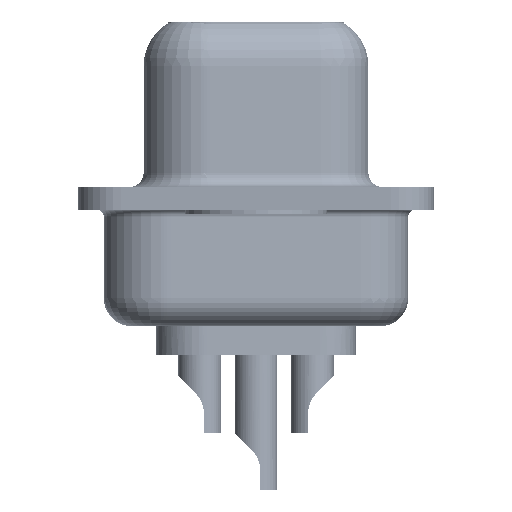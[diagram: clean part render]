
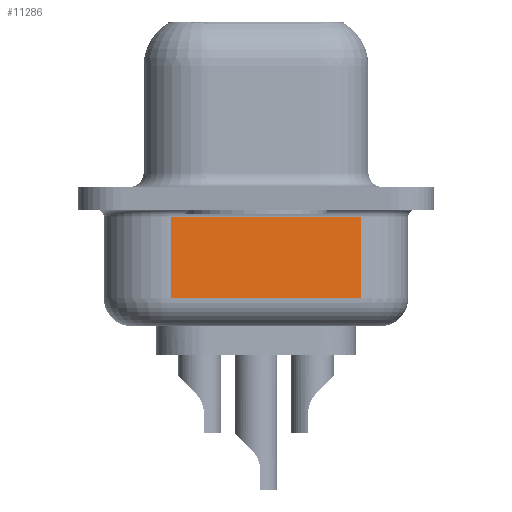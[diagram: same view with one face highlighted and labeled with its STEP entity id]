
A CAD part, left-side view. The second image highlights one B-rep face of the part: STEP entity #11286.
In plain terms, the highlighted planar face has unit normal (-0.985, -0.174, 0).
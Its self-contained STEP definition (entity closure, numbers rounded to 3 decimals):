
#1162 = VERTEX_POINT ( 'NONE', #4410 ) ;
#2598 = CARTESIAN_POINT ( 'NONE',  ( 2.88, 3.003, -4.5 ) ) ;
#3039 = LINE ( 'NONE', #14206, #19122 ) ;
#3407 = VERTEX_POINT ( 'NONE', #22624 ) ;
#4274 = AXIS2_PLACEMENT_3D ( 'NONE', #2598, #13761, #24155 ) ;
#4410 = CARTESIAN_POINT ( 'NONE',  ( 4.062, -3.697, -0.65 ) ) ;
#6225 = DIRECTION ( 'NONE',  ( 0.174, -0.985, 0. ) ) ;
#6767 = ORIENTED_EDGE ( 'NONE', *, *, #7854, .T. ) ;
#7854 = EDGE_CURVE ( 'NONE', #3407, #14603, #31286, .T. ) ;
#8702 = DIRECTION ( 'NONE',  ( 0., 0., 1. ) ) ;
#11286 = ADVANCED_FACE ( 'NONE', ( #21603 ), #35308, .F. ) ;
#12157 = LINE ( 'NONE', #35866, #28927 ) ;
#12516 = CARTESIAN_POINT ( 'NONE',  ( 4.062, -3.697, -3.5 ) ) ;
#13014 = LINE ( 'NONE', #27057, #29633 ) ;
#13237 = VERTEX_POINT ( 'NONE', #25829 ) ;
#13761 = DIRECTION ( 'NONE',  ( 0.985, 0.174, 0. ) ) ;
#14128 = ORIENTED_EDGE ( 'NONE', *, *, #16468, .F. ) ;
#14206 = CARTESIAN_POINT ( 'NONE',  ( 4.062, -3.697, -4.5 ) ) ;
#14603 = VERTEX_POINT ( 'NONE', #12516 ) ;
#14629 = EDGE_CURVE ( 'NONE', #1162, #13237, #12157, .T. ) ;
#16468 = EDGE_CURVE ( 'NONE', #3407, #13237, #13014, .T. ) ;
#19122 = VECTOR ( 'NONE', #8702, 1000. ) ;
#20600 = EDGE_LOOP ( 'NONE', ( #14128, #6767, #32789, #25943 ) ) ;
#21603 = FACE_OUTER_BOUND ( 'NONE', #20600, .T. ) ;
#21624 = DIRECTION ( 'NONE',  ( -0.174, 0.985, 0. ) ) ;
#22624 = CARTESIAN_POINT ( 'NONE',  ( 2.88, 3.003, -3.5 ) ) ;
#24133 = DIRECTION ( 'NONE',  ( 0., 0., 1. ) ) ;
#24155 = DIRECTION ( 'NONE',  ( -0.174, 0.985, 0. ) ) ;
#25751 = EDGE_CURVE ( 'NONE', #14603, #1162, #3039, .T. ) ;
#25829 = CARTESIAN_POINT ( 'NONE',  ( 2.88, 3.003, -0.65 ) ) ;
#25943 = ORIENTED_EDGE ( 'NONE', *, *, #14629, .T. ) ;
#26192 = VECTOR ( 'NONE', #6225, 1000. ) ;
#27057 = CARTESIAN_POINT ( 'NONE',  ( 2.88, 3.003, -4.5 ) ) ;
#28531 = CARTESIAN_POINT ( 'NONE',  ( 2.88, 3.003, -3.5 ) ) ;
#28927 = VECTOR ( 'NONE', #21624, 1000. ) ;
#29633 = VECTOR ( 'NONE', #24133, 1000. ) ;
#31286 = LINE ( 'NONE', #28531, #26192 ) ;
#32789 = ORIENTED_EDGE ( 'NONE', *, *, #25751, .T. ) ;
#35308 = PLANE ( 'NONE',  #4274 ) ;
#35866 = CARTESIAN_POINT ( 'NONE',  ( 2.88, 3.003, -0.65 ) ) ;
